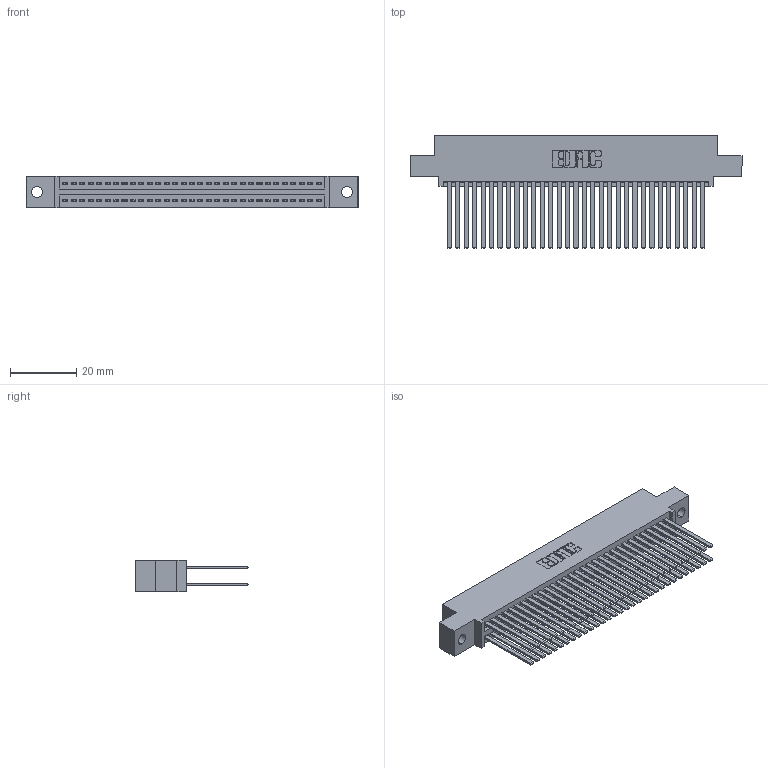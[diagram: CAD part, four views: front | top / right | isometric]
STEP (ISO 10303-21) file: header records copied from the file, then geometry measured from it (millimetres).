
FILE_DESCRIPTION (( 'STEP AP203' ), '1' );
FILE_NAME ('395-062-544-502.STEP', '2019-10-23T16:29:01', ( '' ), ( '' ), 'SwSTEP 2.0', 'SolidWorks 2016', '' );
FILE_SCHEMA (( 'CONFIG_CONTROL_DESIGN' ));
Length unit declared in the file: inch
Products named in the file (3): 395-062-544-502; 345 Part_0.110 Offset - 0.128 Dia; 345-292-001_345-293-144
Assembly tree (63 placements, depth 2):
  395-062-544-502
    345 Part_0.110 Offset - 0.128 Dia
    345-292-001_345-293-144  x62
Bounding box: 99.95 x 33.96 x 9.4 mm (x, y, z)
Volume: 10366.1 mm3; surface area: 17477.3 mm2
Topology: 63 solids, 63 shells, 2858 faces, 8475 edges, 5566 vertices
Faces by surface type: plane 1882, cylinder 976
Entity records: 25755 total; most frequent: CARTESIAN_POINT 4328, ORIENTED_EDGE 4262, DIRECTION 3827, EDGE_CURVE 2131, LINE 1879, VECTOR 1879, VERTEX_POINT 1418, AXIS2_PLACEMENT_3D 974
